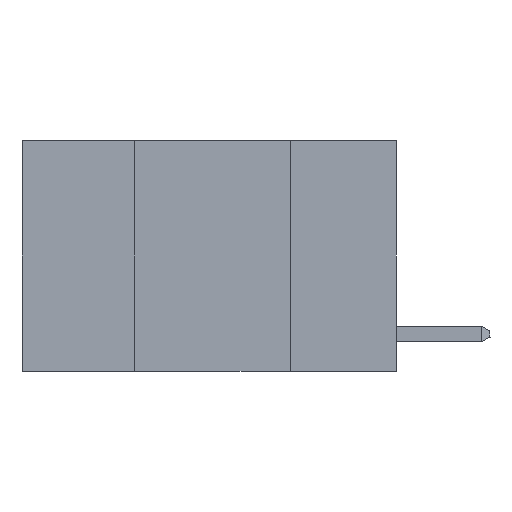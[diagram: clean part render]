
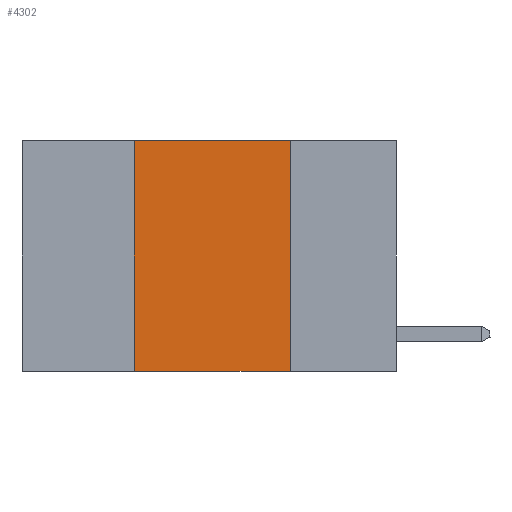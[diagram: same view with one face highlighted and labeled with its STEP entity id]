
A CAD part, left-side view. The second image highlights one B-rep face of the part: STEP entity #4302.
In plain terms, the highlighted planar face has unit normal (-1, 0, 0).
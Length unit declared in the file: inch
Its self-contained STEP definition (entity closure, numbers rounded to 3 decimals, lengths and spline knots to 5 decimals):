
#300 = AXIS2_PLACEMENT_3D ( 'NONE', #8670, #2962, #7874 ) ;
#689 = EDGE_CURVE ( 'NONE', #4054, #3915, #5417, .T. ) ;
#692 = FACE_OUTER_BOUND ( 'NONE', #3851, .T. ) ;
#1137 = CARTESIAN_POINT ( 'NONE',  ( 0., 0.17, 0. ) ) ;
#1214 = CARTESIAN_POINT ( 'NONE',  ( 0., 0.42, 0. ) ) ;
#1394 = EDGE_CURVE ( 'NONE', #9782, #9962, #4726, .T. ) ;
#1994 = LINE ( 'NONE', #1214, #8557 ) ;
#2172 = ORIENTED_EDGE ( 'NONE', *, *, #4629, .F. ) ;
#2525 = CARTESIAN_POINT ( 'NONE',  ( 0., 0.17, 0. ) ) ;
#2562 = CARTESIAN_POINT ( 'NONE',  ( 0., 0.42, 0. ) ) ;
#2810 = VECTOR ( 'NONE', #7841, 39.37008 ) ;
#2962 = DIRECTION ( 'NONE',  ( 1., 0., 0. ) ) ;
#3193 = EDGE_CURVE ( 'NONE', #9962, #3915, #5814, .T. ) ;
#3851 = EDGE_LOOP ( 'NONE', ( #7046, #8485, #2172, #5485 ) ) ;
#3880 = CARTESIAN_POINT ( 'NONE',  ( 0., 0.6, 0. ) ) ;
#3915 = VERTEX_POINT ( 'NONE', #4794 ) ;
#3934 = DIRECTION ( 'NONE',  ( 0., -1., 0. ) ) ;
#4054 = VERTEX_POINT ( 'NONE', #9255 ) ;
#4302 = ADVANCED_FACE ( 'NONE', ( #692 ), #5451, .F. ) ;
#4629 = EDGE_CURVE ( 'NONE', #4054, #9782, #1994, .T. ) ;
#4633 = CARTESIAN_POINT ( 'NONE',  ( 0., 0.6, -0.37 ) ) ;
#4726 = LINE ( 'NONE', #3880, #6232 ) ;
#4794 = CARTESIAN_POINT ( 'NONE',  ( 0., 0.17, -0.37 ) ) ;
#5417 = LINE ( 'NONE', #4633, #2810 ) ;
#5451 = PLANE ( 'NONE',  #300 ) ;
#5485 = ORIENTED_EDGE ( 'NONE', *, *, #689, .T. ) ;
#5764 = DIRECTION ( 'NONE',  ( 0., 0., -1. ) ) ;
#5814 = LINE ( 'NONE', #2525, #8584 ) ;
#6232 = VECTOR ( 'NONE', #3934, 39.37008 ) ;
#7046 = ORIENTED_EDGE ( 'NONE', *, *, #3193, .F. ) ;
#7645 = DIRECTION ( 'NONE',  ( 0., 0., 1. ) ) ;
#7841 = DIRECTION ( 'NONE',  ( 0., -1., 0. ) ) ;
#7874 = DIRECTION ( 'NONE',  ( 0., 0., -1. ) ) ;
#8485 = ORIENTED_EDGE ( 'NONE', *, *, #1394, .F. ) ;
#8557 = VECTOR ( 'NONE', #7645, 39.37008 ) ;
#8584 = VECTOR ( 'NONE', #5764, 39.37008 ) ;
#8670 = CARTESIAN_POINT ( 'NONE',  ( 0., 0.6, 0. ) ) ;
#9255 = CARTESIAN_POINT ( 'NONE',  ( 0., 0.42, -0.37 ) ) ;
#9782 = VERTEX_POINT ( 'NONE', #2562 ) ;
#9962 = VERTEX_POINT ( 'NONE', #1137 ) ;
